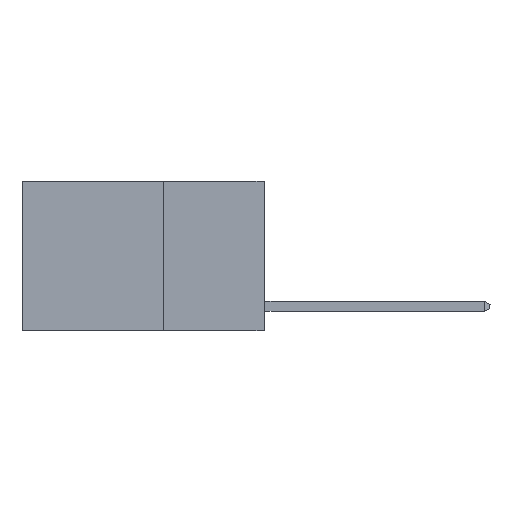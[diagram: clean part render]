
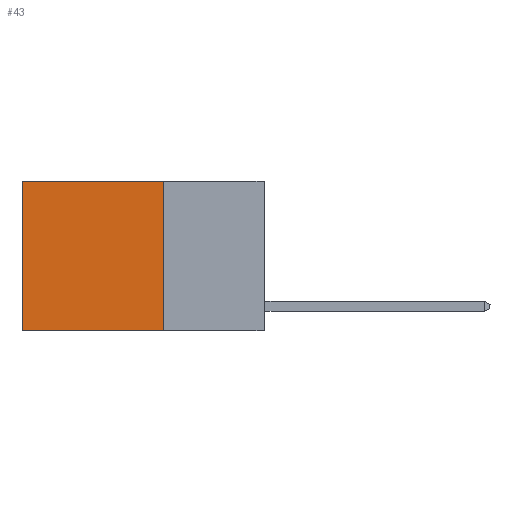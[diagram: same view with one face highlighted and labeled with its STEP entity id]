
A CAD part, left-side view. The second image highlights one B-rep face of the part: STEP entity #43.
In plain terms, the highlighted planar face has unit normal (-1, 0, 0).
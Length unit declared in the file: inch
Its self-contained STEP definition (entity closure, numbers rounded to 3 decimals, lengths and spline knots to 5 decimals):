
#43 = ADVANCED_FACE ( 'NONE', ( #323 ), #10158, .F. ) ;
#57 = AXIS2_PLACEMENT_3D ( 'NONE', #1497, #6583, #1564 ) ;
#323 = FACE_OUTER_BOUND ( 'NONE', #9007, .T. ) ;
#432 = LINE ( 'NONE', #10842, #3017 ) ;
#916 = DIRECTION ( 'NONE',  ( 0., 1., 0. ) ) ;
#1497 = CARTESIAN_POINT ( 'NONE',  ( 0.2625, 0.25, 0. ) ) ;
#1564 = DIRECTION ( 'NONE',  ( 0., 0., -1. ) ) ;
#1889 = CARTESIAN_POINT ( 'NONE',  ( 0.2625, 0.25, -0.37 ) ) ;
#1980 = CARTESIAN_POINT ( 'NONE',  ( 0.2625, 0.25, 0. ) ) ;
#2000 = ORIENTED_EDGE ( 'NONE', *, *, #5511, .T. ) ;
#2296 = ORIENTED_EDGE ( 'NONE', *, *, #6441, .F. ) ;
#2791 = VERTEX_POINT ( 'NONE', #11127 ) ;
#2800 = CARTESIAN_POINT ( 'NONE',  ( 0.2625, 0.25, -0.37 ) ) ;
#3017 = VECTOR ( 'NONE', #9168, 39.37008 ) ;
#4595 = VERTEX_POINT ( 'NONE', #10495 ) ;
#4802 = ORIENTED_EDGE ( 'NONE', *, *, #6356, .T. ) ;
#4937 = EDGE_CURVE ( 'NONE', #6337, #4595, #8769, .T. ) ;
#5511 = EDGE_CURVE ( 'NONE', #2791, #4595, #432, .T. ) ;
#5837 = LINE ( 'NONE', #1980, #10089 ) ;
#6149 = VECTOR ( 'NONE', #7554, 39.37008 ) ;
#6337 = VERTEX_POINT ( 'NONE', #2800 ) ;
#6356 = EDGE_CURVE ( 'NONE', #8182, #2791, #6997, .T. ) ;
#6412 = VECTOR ( 'NONE', #916, 39.37008 ) ;
#6441 = EDGE_CURVE ( 'NONE', #8182, #6337, #5837, .T. ) ;
#6547 = CARTESIAN_POINT ( 'NONE',  ( 0.2625, 0.25, 0. ) ) ;
#6583 = DIRECTION ( 'NONE',  ( 1., 0., 0. ) ) ;
#6997 = LINE ( 'NONE', #11911, #6412 ) ;
#7023 = ORIENTED_EDGE ( 'NONE', *, *, #4937, .F. ) ;
#7554 = DIRECTION ( 'NONE',  ( 0., 1., 0. ) ) ;
#8182 = VERTEX_POINT ( 'NONE', #6547 ) ;
#8583 = DIRECTION ( 'NONE',  ( 0., 0., -1. ) ) ;
#8769 = LINE ( 'NONE', #1889, #6149 ) ;
#9007 = EDGE_LOOP ( 'NONE', ( #2000, #7023, #2296, #4802 ) ) ;
#9168 = DIRECTION ( 'NONE',  ( 0., 0., -1. ) ) ;
#10089 = VECTOR ( 'NONE', #8583, 39.37008 ) ;
#10158 = PLANE ( 'NONE',  #57 ) ;
#10495 = CARTESIAN_POINT ( 'NONE',  ( 0.2625, 0.6, -0.37 ) ) ;
#10842 = CARTESIAN_POINT ( 'NONE',  ( 0.2625, 0.6, 0. ) ) ;
#11127 = CARTESIAN_POINT ( 'NONE',  ( 0.2625, 0.6, 0. ) ) ;
#11911 = CARTESIAN_POINT ( 'NONE',  ( 0.2625, 0.25, 0. ) ) ;
